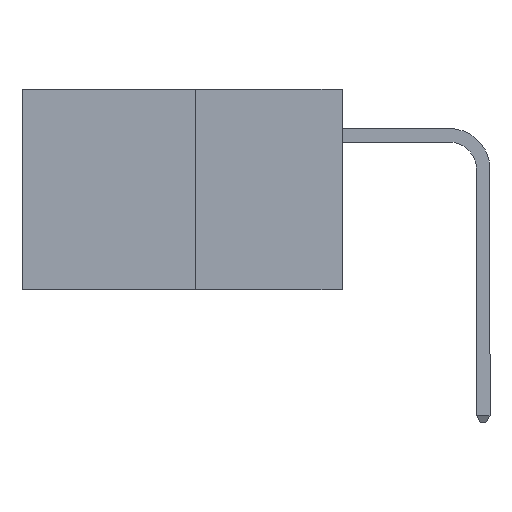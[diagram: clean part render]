
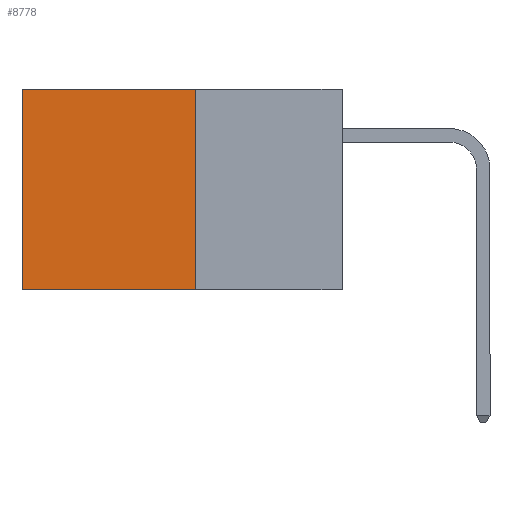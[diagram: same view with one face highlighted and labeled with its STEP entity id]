
A CAD part, left-side view. The second image highlights one B-rep face of the part: STEP entity #8778.
In plain terms, the highlighted planar face has unit normal (-1, 0, 0).
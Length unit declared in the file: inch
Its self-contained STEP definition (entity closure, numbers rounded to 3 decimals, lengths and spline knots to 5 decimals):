
#443 = VERTEX_POINT ( 'NONE', #2235 ) ;
#716 = EDGE_CURVE ( 'NONE', #6204, #1588, #8231, .T. ) ;
#802 = CARTESIAN_POINT ( 'NONE',  ( 0.277, 0.27, 0. ) ) ;
#924 = DIRECTION ( 'NONE',  ( 0., 1., 0. ) ) ;
#1061 = CARTESIAN_POINT ( 'NONE',  ( 0.277, 0.59, -0.37 ) ) ;
#1086 = DIRECTION ( 'NONE',  ( 0., 0., -1. ) ) ;
#1540 = VECTOR ( 'NONE', #924, 39.37008 ) ;
#1588 = VERTEX_POINT ( 'NONE', #6705 ) ;
#1867 = DIRECTION ( 'NONE',  ( 0., 0., -1. ) ) ;
#1912 = LINE ( 'NONE', #802, #3904 ) ;
#2051 = LINE ( 'NONE', #4115, #1540 ) ;
#2235 = CARTESIAN_POINT ( 'NONE',  ( 0.277, 0.59, 0. ) ) ;
#2705 = ORIENTED_EDGE ( 'NONE', *, *, #2869, .F. ) ;
#2836 = DIRECTION ( 'NONE',  ( 0., 0., -1. ) ) ;
#2869 = EDGE_CURVE ( 'NONE', #1588, #5935, #2051, .T. ) ;
#3012 = CARTESIAN_POINT ( 'NONE',  ( 0.277, 0.27, 0. ) ) ;
#3896 = EDGE_CURVE ( 'NONE', #443, #5935, #8612, .T. ) ;
#3904 = VECTOR ( 'NONE', #6832, 39.37008 ) ;
#4079 = AXIS2_PLACEMENT_3D ( 'NONE', #8398, #6335, #1867 ) ;
#4115 = CARTESIAN_POINT ( 'NONE',  ( 0.277, 0.27, -0.37 ) ) ;
#4584 = EDGE_LOOP ( 'NONE', ( #5121, #2705, #9404, #8653 ) ) ;
#4720 = CARTESIAN_POINT ( 'NONE',  ( 0.277, 0.59, -0.37 ) ) ;
#5121 = ORIENTED_EDGE ( 'NONE', *, *, #3896, .T. ) ;
#5596 = PLANE ( 'NONE',  #4079 ) ;
#5874 = CARTESIAN_POINT ( 'NONE',  ( 0.277, 0.27, -0.37 ) ) ;
#5935 = VERTEX_POINT ( 'NONE', #4720 ) ;
#6204 = VERTEX_POINT ( 'NONE', #3012 ) ;
#6335 = DIRECTION ( 'NONE',  ( 1., 0., 0. ) ) ;
#6403 = VECTOR ( 'NONE', #2836, 39.37008 ) ;
#6705 = CARTESIAN_POINT ( 'NONE',  ( 0.277, 0.27, -0.37 ) ) ;
#6832 = DIRECTION ( 'NONE',  ( 0., 1., 0. ) ) ;
#8028 = EDGE_CURVE ( 'NONE', #6204, #443, #1912, .T. ) ;
#8231 = LINE ( 'NONE', #5874, #6403 ) ;
#8385 = FACE_OUTER_BOUND ( 'NONE', #4584, .T. ) ;
#8397 = VECTOR ( 'NONE', #1086, 39.37008 ) ;
#8398 = CARTESIAN_POINT ( 'NONE',  ( 0.277, 0.27, -0.37 ) ) ;
#8612 = LINE ( 'NONE', #1061, #8397 ) ;
#8653 = ORIENTED_EDGE ( 'NONE', *, *, #8028, .T. ) ;
#8778 = ADVANCED_FACE ( 'NONE', ( #8385 ), #5596, .F. ) ;
#9404 = ORIENTED_EDGE ( 'NONE', *, *, #716, .F. ) ;
